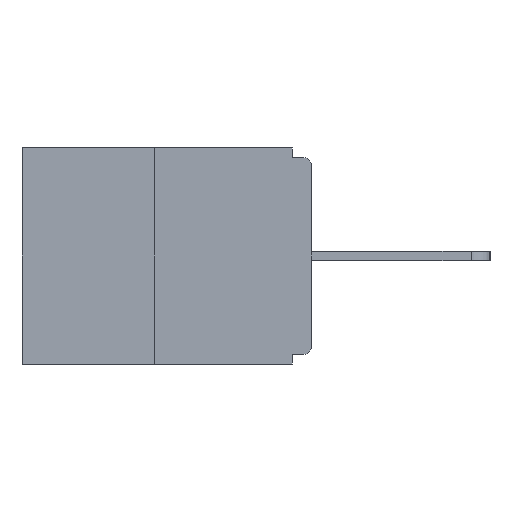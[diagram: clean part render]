
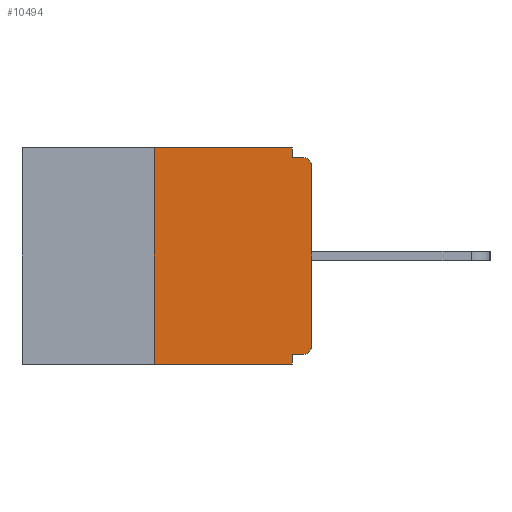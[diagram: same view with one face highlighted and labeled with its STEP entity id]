
A CAD part, left-side view. The second image highlights one B-rep face of the part: STEP entity #10494.
In plain terms, the highlighted planar face has unit normal (-1, 0, 0).
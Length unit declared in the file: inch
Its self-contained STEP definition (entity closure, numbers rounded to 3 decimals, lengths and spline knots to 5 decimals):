
#397 = LINE ( 'NONE', #3539, #15798 ) ;
#668 = LINE ( 'NONE', #4287, #19249 ) ;
#767 = CIRCLE ( 'NONE', #13390, 0.015 ) ;
#1525 = EDGE_CURVE ( 'NONE', #4988, #13385, #7026, .T. ) ;
#1897 = AXIS2_PLACEMENT_3D ( 'NONE', #22813, #7946, #17191 ) ;
#2058 = CARTESIAN_POINT ( 'NONE',  ( 0., 0.015, -0.313 ) ) ;
#2113 = VERTEX_POINT ( 'NONE', #16929 ) ;
#2184 = ORIENTED_EDGE ( 'NONE', *, *, #5531, .F. ) ;
#2300 = EDGE_CURVE ( 'NONE', #4988, #12561, #21358, .T. ) ;
#2602 = DIRECTION ( 'NONE',  ( -1., 0., 0. ) ) ;
#2868 = CARTESIAN_POINT ( 'NONE',  ( 0., 0., 0. ) ) ;
#3265 = VERTEX_POINT ( 'NONE', #20283 ) ;
#3539 = CARTESIAN_POINT ( 'NONE',  ( 0., 0.031, 0. ) ) ;
#3670 = ORIENTED_EDGE ( 'NONE', *, *, #13955, .F. ) ;
#3707 = LINE ( 'NONE', #19632, #4340 ) ;
#3984 = ORIENTED_EDGE ( 'NONE', *, *, #14192, .F. ) ;
#4010 = CARTESIAN_POINT ( 'NONE',  ( 0., 0.25, 0. ) ) ;
#4287 = CARTESIAN_POINT ( 'NONE',  ( 0., 0., -0.328 ) ) ;
#4340 = VECTOR ( 'NONE', #16150, 39.37008 ) ;
#4372 = ORIENTED_EDGE ( 'NONE', *, *, #1525, .T. ) ;
#4988 = VERTEX_POINT ( 'NONE', #8150 ) ;
#4993 = CARTESIAN_POINT ( 'NONE',  ( 0., 0.015, -0.015 ) ) ;
#5211 = VERTEX_POINT ( 'NONE', #18799 ) ;
#5531 = EDGE_CURVE ( 'NONE', #12561, #18305, #22549, .T. ) ;
#5629 = VERTEX_POINT ( 'NONE', #21840 ) ;
#5684 = VERTEX_POINT ( 'NONE', #14759 ) ;
#6216 = DIRECTION ( 'NONE',  ( 0., 0., -1. ) ) ;
#6617 = DIRECTION ( 'NONE',  ( 0., 0., 1. ) ) ;
#6697 = DIRECTION ( 'NONE',  ( 0., 0., 1. ) ) ;
#7026 = LINE ( 'NONE', #14337, #9925 ) ;
#7885 = CIRCLE ( 'NONE', #20150, 0.015 ) ;
#7946 = DIRECTION ( 'NONE',  ( 1., 0., 0. ) ) ;
#8150 = CARTESIAN_POINT ( 'NONE',  ( 0., 0.25, -0.343 ) ) ;
#9925 = VECTOR ( 'NONE', #14452, 39.37008 ) ;
#10022 = ORIENTED_EDGE ( 'NONE', *, *, #15790, .F. ) ;
#10408 = VECTOR ( 'NONE', #6697, 39.37008 ) ;
#10494 = ADVANCED_FACE ( 'NONE', ( #15490 ), #20647, .F. ) ;
#10752 = EDGE_CURVE ( 'NONE', #2113, #5684, #767, .T. ) ;
#11108 = ORIENTED_EDGE ( 'NONE', *, *, #22315, .T. ) ;
#11456 = DIRECTION ( 'NONE',  ( 0., 1., 0. ) ) ;
#12061 = EDGE_CURVE ( 'NONE', #5684, #5211, #21435, .T. ) ;
#12366 = ORIENTED_EDGE ( 'NONE', *, *, #12061, .T. ) ;
#12561 = VERTEX_POINT ( 'NONE', #4010 ) ;
#13342 = ORIENTED_EDGE ( 'NONE', *, *, #17116, .F. ) ;
#13385 = VERTEX_POINT ( 'NONE', #18542 ) ;
#13390 = AXIS2_PLACEMENT_3D ( 'NONE', #2058, #14873, #6216 ) ;
#13955 = EDGE_CURVE ( 'NONE', #2113, #3265, #668, .T. ) ;
#13999 = VECTOR ( 'NONE', #18710, 39.37008 ) ;
#14192 = EDGE_CURVE ( 'NONE', #18305, #5629, #397, .T. ) ;
#14337 = CARTESIAN_POINT ( 'NONE',  ( 0., 0.46, -0.343 ) ) ;
#14452 = DIRECTION ( 'NONE',  ( 0., -1., 0. ) ) ;
#14759 = CARTESIAN_POINT ( 'NONE',  ( 0., 0., -0.313 ) ) ;
#14873 = DIRECTION ( 'NONE',  ( -1., 0., 0. ) ) ;
#15490 = FACE_OUTER_BOUND ( 'NONE', #18665, .T. ) ;
#15652 = CARTESIAN_POINT ( 'NONE',  ( 0., 0., -0.015 ) ) ;
#15790 = EDGE_CURVE ( 'NONE', #5629, #18271, #17585, .T. ) ;
#15798 = VECTOR ( 'NONE', #18617, 39.37008 ) ;
#16150 = DIRECTION ( 'NONE',  ( 0., 0., -1. ) ) ;
#16929 = CARTESIAN_POINT ( 'NONE',  ( 0., 0.015, -0.328 ) ) ;
#17037 = VECTOR ( 'NONE', #21414, 39.37008 ) ;
#17044 = CARTESIAN_POINT ( 'NONE',  ( 0., 0.46, 0. ) ) ;
#17116 = EDGE_CURVE ( 'NONE', #3265, #13385, #3707, .T. ) ;
#17191 = DIRECTION ( 'NONE',  ( 0., 0., -1. ) ) ;
#17585 = LINE ( 'NONE', #15652, #17037 ) ;
#18271 = VERTEX_POINT ( 'NONE', #4993 ) ;
#18305 = VERTEX_POINT ( 'NONE', #21529 ) ;
#18542 = CARTESIAN_POINT ( 'NONE',  ( 0., 0.031, -0.343 ) ) ;
#18617 = DIRECTION ( 'NONE',  ( 0., 0., -1. ) ) ;
#18665 = EDGE_LOOP ( 'NONE', ( #2184, #23462, #4372, #13342, #3670, #20181, #12366, #11108, #10022, #3984 ) ) ;
#18710 = DIRECTION ( 'NONE',  ( 0., -1., 0. ) ) ;
#18799 = CARTESIAN_POINT ( 'NONE',  ( 0., 0., -0.03 ) ) ;
#19006 = CARTESIAN_POINT ( 'NONE',  ( 0., 0.015, -0.03 ) ) ;
#19249 = VECTOR ( 'NONE', #11456, 39.37008 ) ;
#19431 = CARTESIAN_POINT ( 'NONE',  ( 0., 0.25, 0. ) ) ;
#19632 = CARTESIAN_POINT ( 'NONE',  ( 0., 0.031, -0.343 ) ) ;
#20150 = AXIS2_PLACEMENT_3D ( 'NONE', #19006, #2602, #20682 ) ;
#20181 = ORIENTED_EDGE ( 'NONE', *, *, #10752, .T. ) ;
#20283 = CARTESIAN_POINT ( 'NONE',  ( 0., 0.031, -0.328 ) ) ;
#20647 = PLANE ( 'NONE',  #1897 ) ;
#20682 = DIRECTION ( 'NONE',  ( 0., 0., -1. ) ) ;
#21358 = LINE ( 'NONE', #19431, #22092 ) ;
#21414 = DIRECTION ( 'NONE',  ( 0., -1., 0. ) ) ;
#21435 = LINE ( 'NONE', #2868, #10408 ) ;
#21529 = CARTESIAN_POINT ( 'NONE',  ( 0., 0.031, 0. ) ) ;
#21840 = CARTESIAN_POINT ( 'NONE',  ( 0., 0.031, -0.015 ) ) ;
#22092 = VECTOR ( 'NONE', #6617, 39.37008 ) ;
#22315 = EDGE_CURVE ( 'NONE', #5211, #18271, #7885, .T. ) ;
#22549 = LINE ( 'NONE', #17044, #13999 ) ;
#22813 = CARTESIAN_POINT ( 'NONE',  ( 0., 0.46, 0. ) ) ;
#23462 = ORIENTED_EDGE ( 'NONE', *, *, #2300, .F. ) ;
